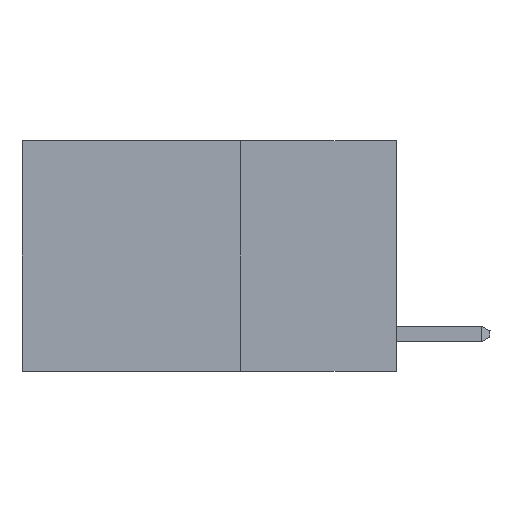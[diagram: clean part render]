
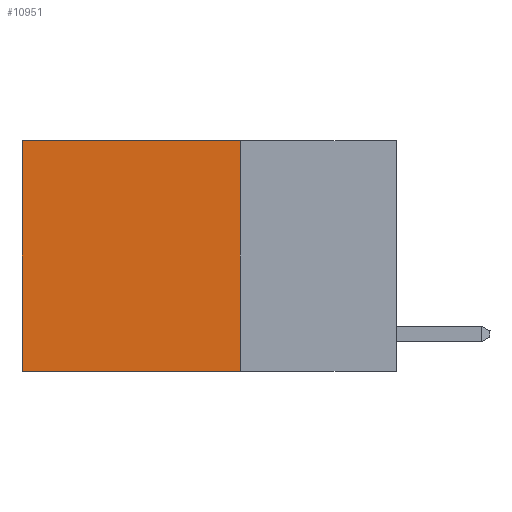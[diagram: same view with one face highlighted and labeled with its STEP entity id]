
A CAD part, left-side view. The second image highlights one B-rep face of the part: STEP entity #10951.
In plain terms, the highlighted planar face has unit normal (-1, 0, 0).
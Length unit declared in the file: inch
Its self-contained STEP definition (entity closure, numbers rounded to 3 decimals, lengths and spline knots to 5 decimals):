
#970 = EDGE_CURVE ( 'NONE', #18397, #13317, #10944, .T. ) ;
#5382 = DIRECTION ( 'NONE',  ( 0., 0., -1. ) ) ;
#6934 = CARTESIAN_POINT ( 'NONE',  ( 0.2625, 0.6, 0. ) ) ;
#8596 = CARTESIAN_POINT ( 'NONE',  ( 0.2625, 0.25, 0. ) ) ;
#9017 = ORIENTED_EDGE ( 'NONE', *, *, #14603, .T. ) ;
#9710 = VECTOR ( 'NONE', #11025, 39.37008 ) ;
#10677 = EDGE_CURVE ( 'NONE', #15316, #23019, #17308, .T. ) ;
#10707 = CARTESIAN_POINT ( 'NONE',  ( 0.2625, 0.25, 0. ) ) ;
#10944 = LINE ( 'NONE', #6934, #9710 ) ;
#10951 = ADVANCED_FACE ( 'NONE', ( #12912 ), #21901, .F. ) ;
#11025 = DIRECTION ( 'NONE',  ( 0., 0., -1. ) ) ;
#12671 = CARTESIAN_POINT ( 'NONE',  ( 0.2625, 0.25, -0.37 ) ) ;
#12912 = FACE_OUTER_BOUND ( 'NONE', #24873, .T. ) ;
#13317 = VERTEX_POINT ( 'NONE', #18972 ) ;
#13824 = LINE ( 'NONE', #12671, #23510 ) ;
#14254 = CARTESIAN_POINT ( 'NONE',  ( 0.2625, 0.25, -0.37 ) ) ;
#14321 = DIRECTION ( 'NONE',  ( 0., 1., 0. ) ) ;
#14603 = EDGE_CURVE ( 'NONE', #15316, #18397, #18777, .T. ) ;
#14638 = DIRECTION ( 'NONE',  ( 0., 1., 0. ) ) ;
#14664 = DIRECTION ( 'NONE',  ( 1., 0., 0. ) ) ;
#15316 = VERTEX_POINT ( 'NONE', #10707 ) ;
#16140 = VECTOR ( 'NONE', #5382, 39.37008 ) ;
#17308 = LINE ( 'NONE', #18897, #16140 ) ;
#18189 = CARTESIAN_POINT ( 'NONE',  ( 0.2625, 0.25, 0. ) ) ;
#18300 = ORIENTED_EDGE ( 'NONE', *, *, #970, .T. ) ;
#18397 = VERTEX_POINT ( 'NONE', #21914 ) ;
#18666 = AXIS2_PLACEMENT_3D ( 'NONE', #18189, #14664, #20479 ) ;
#18777 = LINE ( 'NONE', #8596, #23020 ) ;
#18897 = CARTESIAN_POINT ( 'NONE',  ( 0.2625, 0.25, 0. ) ) ;
#18972 = CARTESIAN_POINT ( 'NONE',  ( 0.2625, 0.6, -0.37 ) ) ;
#19620 = ORIENTED_EDGE ( 'NONE', *, *, #22075, .F. ) ;
#19810 = ORIENTED_EDGE ( 'NONE', *, *, #10677, .F. ) ;
#20479 = DIRECTION ( 'NONE',  ( 0., 0., -1. ) ) ;
#21901 = PLANE ( 'NONE',  #18666 ) ;
#21914 = CARTESIAN_POINT ( 'NONE',  ( 0.2625, 0.6, 0. ) ) ;
#22075 = EDGE_CURVE ( 'NONE', #23019, #13317, #13824, .T. ) ;
#23019 = VERTEX_POINT ( 'NONE', #14254 ) ;
#23020 = VECTOR ( 'NONE', #14321, 39.37008 ) ;
#23510 = VECTOR ( 'NONE', #14638, 39.37008 ) ;
#24873 = EDGE_LOOP ( 'NONE', ( #18300, #19620, #19810, #9017 ) ) ;
